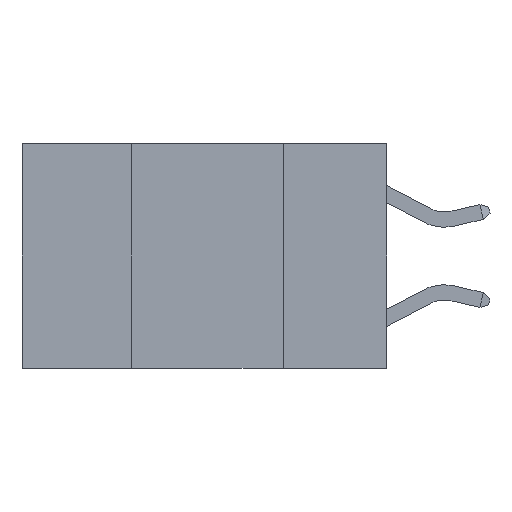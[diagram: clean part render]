
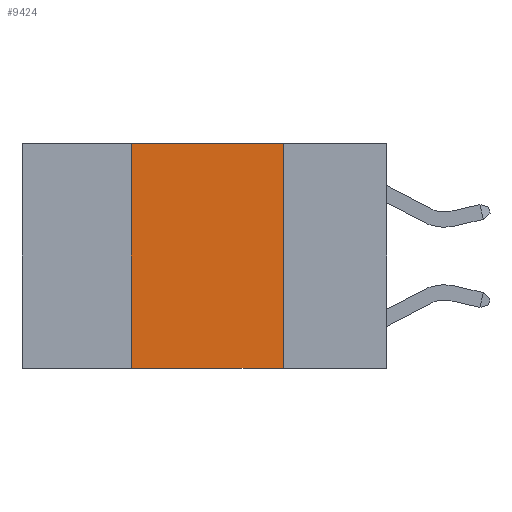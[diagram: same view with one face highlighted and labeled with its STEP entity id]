
A CAD part, left-side view. The second image highlights one B-rep face of the part: STEP entity #9424.
In plain terms, the highlighted planar face has unit normal (-1, 0, 0).
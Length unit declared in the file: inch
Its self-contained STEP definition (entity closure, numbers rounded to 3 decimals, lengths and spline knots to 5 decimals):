
#176 = CARTESIAN_POINT ( 'NONE',  ( 0., 0.6, -0.37 ) ) ;
#180 = LINE ( 'NONE', #2334, #4344 ) ;
#765 = VERTEX_POINT ( 'NONE', #9470 ) ;
#812 = LINE ( 'NONE', #7252, #7173 ) ;
#1338 = ORIENTED_EDGE ( 'NONE', *, *, #3629, .F. ) ;
#2334 = CARTESIAN_POINT ( 'NONE',  ( 0., 0.42, 0. ) ) ;
#2502 = DIRECTION ( 'NONE',  ( 1., 0., 0. ) ) ;
#3520 = CARTESIAN_POINT ( 'NONE',  ( 0., 0.42, 0. ) ) ;
#3629 = EDGE_CURVE ( 'NONE', #8897, #5764, #812, .T. ) ;
#3653 = CARTESIAN_POINT ( 'NONE',  ( 0., 0.17, 0. ) ) ;
#3752 = DIRECTION ( 'NONE',  ( 0., 0., 1. ) ) ;
#3805 = EDGE_CURVE ( 'NONE', #5112, #8897, #180, .T. ) ;
#3848 = EDGE_CURVE ( 'NONE', #5764, #765, #7900, .T. ) ;
#3906 = EDGE_CURVE ( 'NONE', #5112, #765, #7160, .T. ) ;
#3908 = FACE_OUTER_BOUND ( 'NONE', #4951, .T. ) ;
#3944 = ORIENTED_EDGE ( 'NONE', *, *, #3805, .F. ) ;
#4344 = VECTOR ( 'NONE', #3752, 39.37008 ) ;
#4455 = DIRECTION ( 'NONE',  ( 0., -1., 0. ) ) ;
#4951 = EDGE_LOOP ( 'NONE', ( #8584, #1338, #3944, #8500 ) ) ;
#5112 = VERTEX_POINT ( 'NONE', #6575 ) ;
#5764 = VERTEX_POINT ( 'NONE', #9228 ) ;
#5780 = VECTOR ( 'NONE', #9334, 39.37008 ) ;
#6575 = CARTESIAN_POINT ( 'NONE',  ( 0., 0.42, -0.37 ) ) ;
#7160 = LINE ( 'NONE', #176, #9127 ) ;
#7173 = VECTOR ( 'NONE', #8284, 39.37008 ) ;
#7252 = CARTESIAN_POINT ( 'NONE',  ( 0., 0.6, 0. ) ) ;
#7494 = PLANE ( 'NONE',  #10338 ) ;
#7900 = LINE ( 'NONE', #3653, #5780 ) ;
#8284 = DIRECTION ( 'NONE',  ( 0., -1., 0. ) ) ;
#8302 = DIRECTION ( 'NONE',  ( 0., 0., -1. ) ) ;
#8500 = ORIENTED_EDGE ( 'NONE', *, *, #3906, .T. ) ;
#8584 = ORIENTED_EDGE ( 'NONE', *, *, #3848, .F. ) ;
#8897 = VERTEX_POINT ( 'NONE', #3520 ) ;
#9127 = VECTOR ( 'NONE', #4455, 39.37008 ) ;
#9228 = CARTESIAN_POINT ( 'NONE',  ( 0., 0.17, 0. ) ) ;
#9334 = DIRECTION ( 'NONE',  ( 0., 0., -1. ) ) ;
#9424 = ADVANCED_FACE ( 'NONE', ( #3908 ), #7494, .F. ) ;
#9470 = CARTESIAN_POINT ( 'NONE',  ( 0., 0.17, -0.37 ) ) ;
#10016 = CARTESIAN_POINT ( 'NONE',  ( 0., 0.6, 0. ) ) ;
#10338 = AXIS2_PLACEMENT_3D ( 'NONE', #10016, #2502, #8302 ) ;
